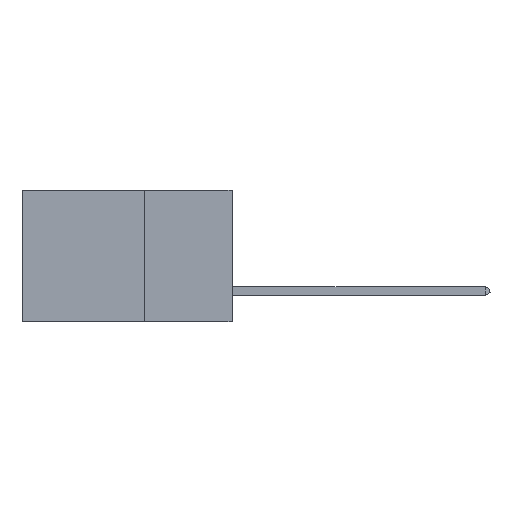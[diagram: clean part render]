
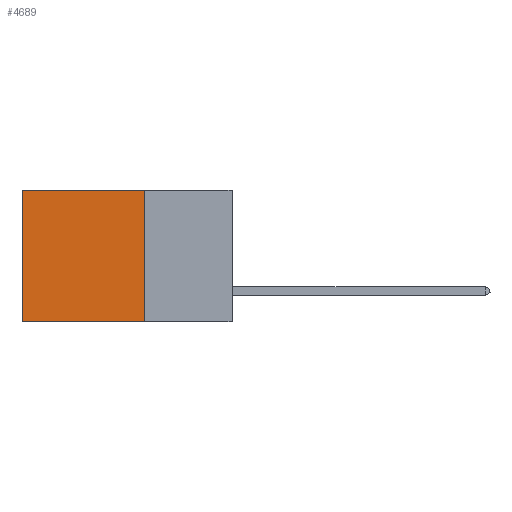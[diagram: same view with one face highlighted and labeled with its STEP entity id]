
A CAD part, left-side view. The second image highlights one B-rep face of the part: STEP entity #4689.
In plain terms, the highlighted planar face has unit normal (-1, 0, 0).
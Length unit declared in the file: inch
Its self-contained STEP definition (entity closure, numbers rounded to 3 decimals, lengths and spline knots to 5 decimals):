
#132 = CARTESIAN_POINT ( 'NONE',  ( 0.2875, 0.25, 0. ) ) ;
#455 = ORIENTED_EDGE ( 'NONE', *, *, #4800, .T. ) ;
#867 = CARTESIAN_POINT ( 'NONE',  ( 0.2875, 0.6, -0.375 ) ) ;
#1271 = PLANE ( 'NONE',  #12589 ) ;
#1936 = VECTOR ( 'NONE', #10211, 39.37008 ) ;
#2137 = ORIENTED_EDGE ( 'NONE', *, *, #5057, .T. ) ;
#2508 = VERTEX_POINT ( 'NONE', #15564 ) ;
#2577 = VERTEX_POINT ( 'NONE', #11586 ) ;
#3239 = CARTESIAN_POINT ( 'NONE',  ( 0.2875, 0.25, -0.375 ) ) ;
#3284 = VERTEX_POINT ( 'NONE', #9208 ) ;
#3452 = VECTOR ( 'NONE', #16632, 39.37008 ) ;
#4136 = LINE ( 'NONE', #8456, #10984 ) ;
#4332 = FACE_OUTER_BOUND ( 'NONE', #17076, .T. ) ;
#4689 = ADVANCED_FACE ( 'NONE', ( #4332 ), #1271, .F. ) ;
#4800 = EDGE_CURVE ( 'NONE', #11342, #3284, #6213, .T. ) ;
#5057 = EDGE_CURVE ( 'NONE', #3284, #2577, #13491, .T. ) ;
#5263 = LINE ( 'NONE', #3239, #6790 ) ;
#6032 = DIRECTION ( 'NONE',  ( 0., 0., -1. ) ) ;
#6213 = LINE ( 'NONE', #132, #3452 ) ;
#6786 = CARTESIAN_POINT ( 'NONE',  ( 0.2875, 0.25, -0.375 ) ) ;
#6790 = VECTOR ( 'NONE', #6032, 39.37008 ) ;
#7443 = CARTESIAN_POINT ( 'NONE',  ( 0.2875, 0.25, 0. ) ) ;
#8456 = CARTESIAN_POINT ( 'NONE',  ( 0.2875, 0.25, -0.375 ) ) ;
#8853 = EDGE_CURVE ( 'NONE', #2508, #2577, #4136, .T. ) ;
#9208 = CARTESIAN_POINT ( 'NONE',  ( 0.2875, 0.6, 0. ) ) ;
#9530 = DIRECTION ( 'NONE',  ( 0., 0., -1. ) ) ;
#10211 = DIRECTION ( 'NONE',  ( 0., 0., -1. ) ) ;
#10984 = VECTOR ( 'NONE', #16479, 39.37008 ) ;
#11342 = VERTEX_POINT ( 'NONE', #7443 ) ;
#11586 = CARTESIAN_POINT ( 'NONE',  ( 0.2875, 0.6, -0.375 ) ) ;
#11646 = ORIENTED_EDGE ( 'NONE', *, *, #17389, .F. ) ;
#12589 = AXIS2_PLACEMENT_3D ( 'NONE', #6786, #17795, #9530 ) ;
#13491 = LINE ( 'NONE', #867, #1936 ) ;
#14885 = ORIENTED_EDGE ( 'NONE', *, *, #8853, .F. ) ;
#15564 = CARTESIAN_POINT ( 'NONE',  ( 0.2875, 0.25, -0.375 ) ) ;
#16479 = DIRECTION ( 'NONE',  ( 0., 1., 0. ) ) ;
#16632 = DIRECTION ( 'NONE',  ( 0., 1., 0. ) ) ;
#17076 = EDGE_LOOP ( 'NONE', ( #2137, #14885, #11646, #455 ) ) ;
#17389 = EDGE_CURVE ( 'NONE', #11342, #2508, #5263, .T. ) ;
#17795 = DIRECTION ( 'NONE',  ( 1., 0., 0. ) ) ;
